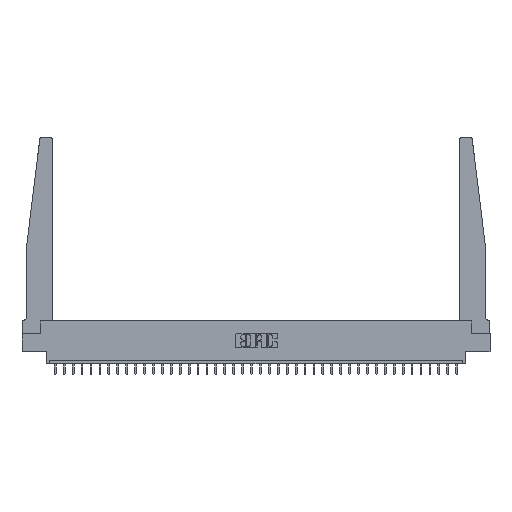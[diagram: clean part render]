
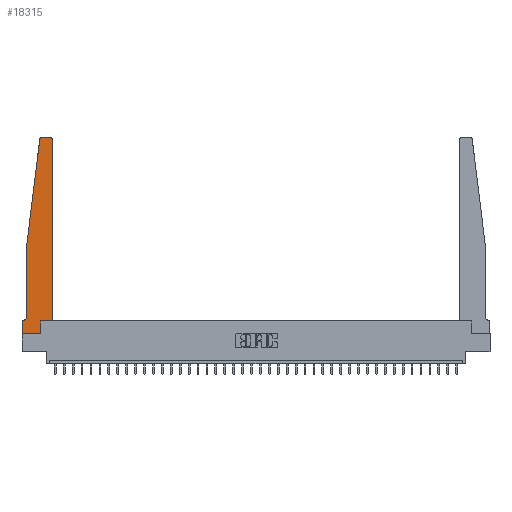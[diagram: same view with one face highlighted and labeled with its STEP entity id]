
A CAD part, top view. The second image highlights one B-rep face of the part: STEP entity #18315.
In plain terms, the highlighted planar face has unit normal (0, 0, 1).
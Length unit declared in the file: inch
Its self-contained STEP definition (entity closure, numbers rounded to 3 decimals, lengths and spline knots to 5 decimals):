
#115 = CARTESIAN_POINT ( 'NONE',  ( 0.065, 1.25, 0.37 ) ) ;
#422 = CARTESIAN_POINT ( 'NONE',  ( 0.065, 0.2375, 0.37 ) ) ;
#1460 = EDGE_CURVE ( 'NONE', #25365, #17660, #26171, .T. ) ;
#1729 = VECTOR ( 'NONE', #4439, 39.37008 ) ;
#1805 = ORIENTED_EDGE ( 'NONE', *, *, #32449, .T. ) ;
#1875 = VECTOR ( 'NONE', #14399, 39.37008 ) ;
#2166 = CARTESIAN_POINT ( 'NONE',  ( 0.425, 2.72, 0.37 ) ) ;
#2439 = ORIENTED_EDGE ( 'NONE', *, *, #21810, .T. ) ;
#2994 = CARTESIAN_POINT ( 'NONE',  ( 0., 0., 0.37 ) ) ;
#3490 = VECTOR ( 'NONE', #13999, 39.37008 ) ;
#3839 = CARTESIAN_POINT ( 'NONE',  ( 0.2605, 0.18, 0.37 ) ) ;
#3957 = ORIENTED_EDGE ( 'NONE', *, *, #32327, .T. ) ;
#4068 = AXIS2_PLACEMENT_3D ( 'NONE', #16771, #13355, #11830 ) ;
#4107 = ORIENTED_EDGE ( 'NONE', *, *, #31638, .T. ) ;
#4133 = EDGE_LOOP ( 'NONE', ( #32457, #4170, #30086, #1805, #21377, #20184, #3957, #4155, #4107, #2439, #8281, #15044 ) ) ;
#4155 = ORIENTED_EDGE ( 'NONE', *, *, #20861, .T. ) ;
#4170 = ORIENTED_EDGE ( 'NONE', *, *, #13717, .T. ) ;
#4439 = DIRECTION ( 'NONE',  ( 0., 1., 0. ) ) ;
#4517 = VERTEX_POINT ( 'NONE', #17248 ) ;
#5262 = DIRECTION ( 'NONE',  ( 0., 0., 1. ) ) ;
#5455 = CARTESIAN_POINT ( 'NONE',  ( 0.27653, 2.75, 0.37 ) ) ;
#5489 = CIRCLE ( 'NONE', #6367, 0.05 ) ;
#5916 = VERTEX_POINT ( 'NONE', #115 ) ;
#6014 = CARTESIAN_POINT ( 'NONE',  ( 0.24675, 2.72367, 0.37 ) ) ;
#6160 = VECTOR ( 'NONE', #18480, 39.37008 ) ;
#6367 = AXIS2_PLACEMENT_3D ( 'NONE', #27859, #12647, #15218 ) ;
#6716 = CARTESIAN_POINT ( 'NONE',  ( 0., 0., 0.37 ) ) ;
#7606 = CARTESIAN_POINT ( 'NONE',  ( 0.2605, 0.18, 0.37 ) ) ;
#7854 = LINE ( 'NONE', #3839, #3490 ) ;
#7973 = DIRECTION ( 'NONE',  ( 1., 0., 0. ) ) ;
#8253 = DIRECTION ( 'NONE',  ( 1., 0., 0. ) ) ;
#8281 = ORIENTED_EDGE ( 'NONE', *, *, #15927, .T. ) ;
#8572 = VERTEX_POINT ( 'NONE', #15713 ) ;
#10396 = VERTEX_POINT ( 'NONE', #29100 ) ;
#10923 = DIRECTION ( 'NONE',  ( -1., 0., 0. ) ) ;
#10993 = VECTOR ( 'NONE', #17613, 39.37008 ) ;
#11456 = VERTEX_POINT ( 'NONE', #2166 ) ;
#11721 = EDGE_CURVE ( 'NONE', #11456, #25365, #22443, .T. ) ;
#11830 = DIRECTION ( 'NONE',  ( 1., 0., 0. ) ) ;
#11938 = CIRCLE ( 'NONE', #20346, 0.03 ) ;
#12032 = EDGE_CURVE ( 'NONE', #29714, #5916, #30339, .T. ) ;
#12647 = DIRECTION ( 'NONE',  ( 0., 0., -1. ) ) ;
#12915 = LINE ( 'NONE', #22759, #32392 ) ;
#12957 = CARTESIAN_POINT ( 'NONE',  ( 0.27653, 2.72, 0.37 ) ) ;
#13355 = DIRECTION ( 'NONE',  ( 0., 0., 1. ) ) ;
#13391 = LINE ( 'NONE', #2994, #6160 ) ;
#13717 = EDGE_CURVE ( 'NONE', #17660, #29714, #11938, .T. ) ;
#13999 = DIRECTION ( 'NONE',  ( 0., 1., 0. ) ) ;
#14399 = DIRECTION ( 'NONE',  ( 0., -1., 0. ) ) ;
#14701 = FACE_OUTER_BOUND ( 'NONE', #4133, .T. ) ;
#14861 = AXIS2_PLACEMENT_3D ( 'NONE', #28752, #21142, #7973 ) ;
#15044 = ORIENTED_EDGE ( 'NONE', *, *, #11721, .T. ) ;
#15085 = LINE ( 'NONE', #18474, #24628 ) ;
#15218 = DIRECTION ( 'NONE',  ( -1., 0., 0. ) ) ;
#15713 = CARTESIAN_POINT ( 'NONE',  ( 0., 0.1875, 0.37 ) ) ;
#15927 = EDGE_CURVE ( 'NONE', #23994, #11456, #20041, .T. ) ;
#16771 = CARTESIAN_POINT ( 'NONE',  ( 0.395, 2.72, 0.37 ) ) ;
#17248 = CARTESIAN_POINT ( 'NONE',  ( 0., 0., 0.37 ) ) ;
#17359 = CARTESIAN_POINT ( 'NONE',  ( 0.425, 0.18, 0.37 ) ) ;
#17613 = DIRECTION ( 'NONE',  ( 0., -1., 0. ) ) ;
#17660 = VERTEX_POINT ( 'NONE', #5455 ) ;
#18315 = ADVANCED_FACE ( 'NONE', ( #14701 ), #18568, .T. ) ;
#18474 = CARTESIAN_POINT ( 'NONE',  ( 0.065, 0.1875, 0.37 ) ) ;
#18480 = DIRECTION ( 'NONE',  ( 1., 0., 0. ) ) ;
#18568 = PLANE ( 'NONE',  #14861 ) ;
#20041 = LINE ( 'NONE', #17359, #1729 ) ;
#20184 = ORIENTED_EDGE ( 'NONE', *, *, #27650, .T. ) ;
#20191 = LINE ( 'NONE', #6716, #1875 ) ;
#20346 = AXIS2_PLACEMENT_3D ( 'NONE', #12957, #5262, #8253 ) ;
#20861 = EDGE_CURVE ( 'NONE', #4517, #10396, #13391, .T. ) ;
#21142 = DIRECTION ( 'NONE',  ( 0., 0., 1. ) ) ;
#21377 = ORIENTED_EDGE ( 'NONE', *, *, #28057, .T. ) ;
#21810 = EDGE_CURVE ( 'NONE', #22814, #23994, #12915, .T. ) ;
#21820 = VECTOR ( 'NONE', #10923, 39.37008 ) ;
#22439 = DIRECTION ( 'NONE',  ( 1., 0., 0. ) ) ;
#22443 = CIRCLE ( 'NONE', #4068, 0.03 ) ;
#22708 = VERTEX_POINT ( 'NONE', #422 ) ;
#22759 = CARTESIAN_POINT ( 'NONE',  ( 0.425, 0.18, 0.37 ) ) ;
#22814 = VERTEX_POINT ( 'NONE', #7606 ) ;
#23286 = CARTESIAN_POINT ( 'NONE',  ( 0.395, 2.75, 0.37 ) ) ;
#23994 = VERTEX_POINT ( 'NONE', #25574 ) ;
#24628 = VECTOR ( 'NONE', #31021, 39.37008 ) ;
#25365 = VERTEX_POINT ( 'NONE', #23286 ) ;
#25574 = CARTESIAN_POINT ( 'NONE',  ( 0.425, 0.18, 0.37 ) ) ;
#26171 = LINE ( 'NONE', #30829, #21820 ) ;
#26596 = CARTESIAN_POINT ( 'NONE',  ( 0.065, 1.25, 0.37 ) ) ;
#27515 = VERTEX_POINT ( 'NONE', #28004 ) ;
#27650 = EDGE_CURVE ( 'NONE', #27515, #8572, #15085, .T. ) ;
#27859 = CARTESIAN_POINT ( 'NONE',  ( 0.015, 0.2375, 0.37 ) ) ;
#28004 = CARTESIAN_POINT ( 'NONE',  ( 0.015, 0.1875, 0.37 ) ) ;
#28057 = EDGE_CURVE ( 'NONE', #22708, #27515, #5489, .T. ) ;
#28752 = CARTESIAN_POINT ( 'NONE',  ( 0., 0.1875, 0.37 ) ) ;
#29100 = CARTESIAN_POINT ( 'NONE',  ( 0.2605, 0., 0.37 ) ) ;
#29131 = DIRECTION ( 'NONE',  ( -0.122, -0.992, 0. ) ) ;
#29714 = VERTEX_POINT ( 'NONE', #6014 ) ;
#30086 = ORIENTED_EDGE ( 'NONE', *, *, #12032, .T. ) ;
#30339 = LINE ( 'NONE', #26596, #30736 ) ;
#30584 = CARTESIAN_POINT ( 'NONE',  ( 0.065, 1.25, 0.37 ) ) ;
#30736 = VECTOR ( 'NONE', #29131, 39.37008 ) ;
#30829 = CARTESIAN_POINT ( 'NONE',  ( 0.25, 2.75, 0.37 ) ) ;
#30868 = LINE ( 'NONE', #30584, #10993 ) ;
#31021 = DIRECTION ( 'NONE',  ( -1., 0., 0. ) ) ;
#31638 = EDGE_CURVE ( 'NONE', #10396, #22814, #7854, .T. ) ;
#32327 = EDGE_CURVE ( 'NONE', #8572, #4517, #20191, .T. ) ;
#32392 = VECTOR ( 'NONE', #22439, 39.37008 ) ;
#32449 = EDGE_CURVE ( 'NONE', #5916, #22708, #30868, .T. ) ;
#32457 = ORIENTED_EDGE ( 'NONE', *, *, #1460, .T. ) ;
